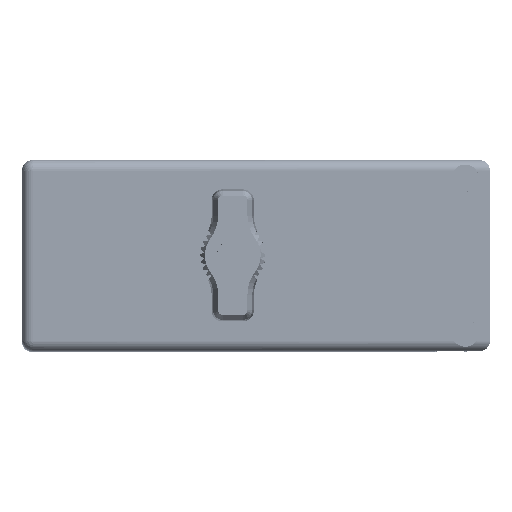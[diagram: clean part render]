
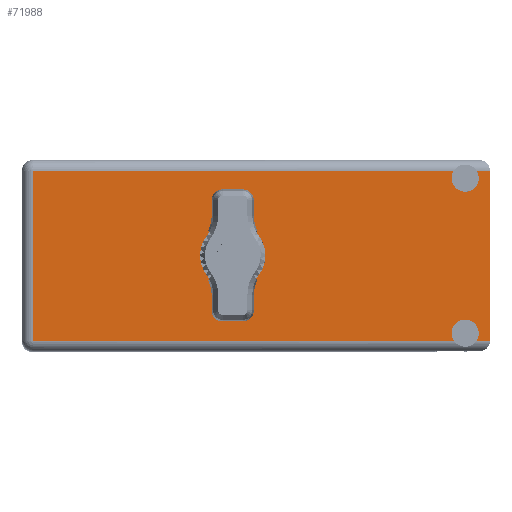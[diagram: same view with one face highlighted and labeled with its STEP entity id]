
A CAD part, top view. The second image highlights one B-rep face of the part: STEP entity #71988.
In plain terms, the highlighted face is planar.
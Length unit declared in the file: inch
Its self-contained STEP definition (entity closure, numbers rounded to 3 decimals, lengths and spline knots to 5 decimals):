
#157 = DIRECTION ( 'NONE',  ( -1., 0., 0. ) ) ;
#240 = AXIS2_PLACEMENT_3D ( 'NONE', #29537, #90201, #157 ) ;
#545 = EDGE_CURVE ( 'NONE', #49202, #39092, #40444, .T. ) ;
#742 = CIRCLE ( 'NONE', #60126, 0.125 ) ;
#1376 = LINE ( 'NONE', #47346, #81972 ) ;
#2965 = ORIENTED_EDGE ( 'NONE', *, *, #45895, .F. ) ;
#4074 = ORIENTED_EDGE ( 'NONE', *, *, #80457, .F. ) ;
#6186 = CARTESIAN_POINT ( 'NONE',  ( 0., 1.675, 0. ) ) ;
#7179 = DIRECTION ( 'NONE',  ( 0., 0., 1. ) ) ;
#8169 = LINE ( 'NONE', #76158, #36929 ) ;
#8355 = DIRECTION ( 'NONE',  ( 0., 0., 1. ) ) ;
#8837 = CARTESIAN_POINT ( 'NONE',  ( 1.499, 1.675, 0.5 ) ) ;
#9008 = VERTEX_POINT ( 'NONE', #22564 ) ;
#10022 = EDGE_CURVE ( 'NONE', #57169, #67750, #8169, .T. ) ;
#12033 = VERTEX_POINT ( 'NONE', #65398 ) ;
#13999 = CARTESIAN_POINT ( 'NONE',  ( -1.359, 1.675, -0.547 ) ) ;
#14849 = FACE_OUTER_BOUND ( 'NONE', #69428, .T. ) ;
#14934 = ORIENTED_EDGE ( 'NONE', *, *, #545, .F. ) ;
#15475 = DIRECTION ( 'NONE',  ( -1., 0., 0. ) ) ;
#17427 = ORIENTED_EDGE ( 'NONE', *, *, #10022, .T. ) ;
#17647 = VERTEX_POINT ( 'NONE', #90620 ) ;
#18313 = LINE ( 'NONE', #78057, #55461 ) ;
#19365 = EDGE_CURVE ( 'NONE', #66767, #9008, #59219, .T. ) ;
#20354 = DIRECTION ( 'NONE',  ( 0., 0., 1. ) ) ;
#22233 = AXIS2_PLACEMENT_3D ( 'NONE', #75167, #61411, #7179 ) ;
#22564 = CARTESIAN_POINT ( 'NONE',  ( -1.289, 1.675, 0.547 ) ) ;
#22662 = FACE_BOUND ( 'NONE', #23826, .T. ) ;
#23826 = EDGE_LOOP ( 'NONE', ( #58635, #71848 ) ) ;
#25578 = CARTESIAN_POINT ( 'NONE',  ( 1.57281, 1.675, -0.547 ) ) ;
#27305 = EDGE_CURVE ( 'NONE', #12033, #66767, #95236, .T. ) ;
#27334 = EDGE_CURVE ( 'NONE', #17647, #52103, #742, .T. ) ;
#27689 = EDGE_CURVE ( 'NONE', #52103, #17647, #45992, .T. ) ;
#27921 = DIRECTION ( 'NONE',  ( 0., 0., 1. ) ) ;
#28502 = DIRECTION ( 'NONE',  ( 0., 1., 0. ) ) ;
#29537 = CARTESIAN_POINT ( 'NONE',  ( -1.359, 1.675, -0.617 ) ) ;
#33603 = CARTESIAN_POINT ( 'NONE',  ( 1.57281, 1.675, 0.547 ) ) ;
#36219 = CARTESIAN_POINT ( 'NONE',  ( 1.499, 1.675, -0.5 ) ) ;
#36795 = CARTESIAN_POINT ( 'NONE',  ( 1.499, 1.675, 0.5 ) ) ;
#36929 = VECTOR ( 'NONE', #15475, 39.37008 ) ;
#36974 = ORIENTED_EDGE ( 'NONE', *, *, #95098, .F. ) ;
#38511 = EDGE_CURVE ( 'NONE', #58646, #67750, #48663, .T. ) ;
#38644 = DIRECTION ( 'NONE',  ( 0., 1., 0. ) ) ;
#39092 = VERTEX_POINT ( 'NONE', #65973 ) ;
#40444 = CIRCLE ( 'NONE', #96788, 0.0875 ) ;
#41297 = AXIS2_PLACEMENT_3D ( 'NONE', #59632, #66966, #52278 ) ;
#41910 = CARTESIAN_POINT ( 'NONE',  ( 1.499, 1.675, -0.4125 ) ) ;
#43825 = DIRECTION ( 'NONE',  ( -1., 0., 0. ) ) ;
#45895 = EDGE_CURVE ( 'NONE', #57169, #48345, #94169, .T. ) ;
#45992 = CIRCLE ( 'NONE', #41297, 0.125 ) ;
#46179 = ORIENTED_EDGE ( 'NONE', *, *, #19365, .T. ) ;
#46536 = EDGE_CURVE ( 'NONE', #56596, #48345, #1376, .T. ) ;
#47346 = CARTESIAN_POINT ( 'NONE',  ( 1.659, 1.675, 0.547 ) ) ;
#48345 = VERTEX_POINT ( 'NONE', #94891 ) ;
#48663 = CIRCLE ( 'NONE', #64315, 0.0875 ) ;
#48972 = EDGE_CURVE ( 'NONE', #9008, #39092, #18313, .T. ) ;
#49202 = VERTEX_POINT ( 'NONE', #73497 ) ;
#50108 = CARTESIAN_POINT ( 'NONE',  ( 0., 1.675, 0.125 ) ) ;
#51509 = ORIENTED_EDGE ( 'NONE', *, *, #27305, .T. ) ;
#52103 = VERTEX_POINT ( 'NONE', #50108 ) ;
#52278 = DIRECTION ( 'NONE',  ( 0., 0., 1. ) ) ;
#53714 = AXIS2_PLACEMENT_3D ( 'NONE', #8837, #38644, #8355 ) ;
#55461 = VECTOR ( 'NONE', #61912, 39.37008 ) ;
#56596 = VERTEX_POINT ( 'NONE', #33603 ) ;
#57169 = VERTEX_POINT ( 'NONE', #80468 ) ;
#58635 = ORIENTED_EDGE ( 'NONE', *, *, #27689, .F. ) ;
#58646 = VERTEX_POINT ( 'NONE', #41910 ) ;
#59219 = LINE ( 'NONE', #89082, #67057 ) ;
#59632 = CARTESIAN_POINT ( 'NONE',  ( 0., 1.675, 0. ) ) ;
#60126 = AXIS2_PLACEMENT_3D ( 'NONE', #6186, #96690, #20354 ) ;
#61411 = DIRECTION ( 'NONE',  ( 0., 1., 0. ) ) ;
#61912 = DIRECTION ( 'NONE',  ( 1., 0., 0. ) ) ;
#62518 = DIRECTION ( 'NONE',  ( 1., 0., 0. ) ) ;
#63637 = VECTOR ( 'NONE', #65753, 39.37008 ) ;
#64315 = AXIS2_PLACEMENT_3D ( 'NONE', #36219, #86667, #71985 ) ;
#65398 = CARTESIAN_POINT ( 'NONE',  ( 1.42519, 1.675, -0.547 ) ) ;
#65753 = DIRECTION ( 'NONE',  ( 0., 0., 1. ) ) ;
#65973 = CARTESIAN_POINT ( 'NONE',  ( 1.42519, 1.675, 0.547 ) ) ;
#66649 = DIRECTION ( 'NONE',  ( 0., 0., 1. ) ) ;
#66716 = PLANE ( 'NONE',  #240 ) ;
#66767 = VERTEX_POINT ( 'NONE', #85494 ) ;
#66966 = DIRECTION ( 'NONE',  ( 0., 1., 0. ) ) ;
#67057 = VECTOR ( 'NONE', #27921, 39.37008 ) ;
#67750 = VERTEX_POINT ( 'NONE', #25578 ) ;
#69428 = EDGE_LOOP ( 'NONE', ( #77994, #14934, #36974, #83985, #2965, #17427, #95449, #4074, #51509, #46179 ) ) ;
#70895 = CIRCLE ( 'NONE', #53714, 0.0875 ) ;
#71848 = ORIENTED_EDGE ( 'NONE', *, *, #27334, .F. ) ;
#71985 = DIRECTION ( 'NONE',  ( 0., 0., 1. ) ) ;
#71988 = ADVANCED_FACE ( 'NONE', ( #22662, #14849 ), #66716, .T. ) ;
#73497 = CARTESIAN_POINT ( 'NONE',  ( 1.499, 1.675, 0.4125 ) ) ;
#75167 = CARTESIAN_POINT ( 'NONE',  ( 1.499, 1.675, -0.5 ) ) ;
#75718 = VECTOR ( 'NONE', #43825, 39.37008 ) ;
#76158 = CARTESIAN_POINT ( 'NONE',  ( -1.359, 1.675, -0.547 ) ) ;
#77994 = ORIENTED_EDGE ( 'NONE', *, *, #48972, .T. ) ;
#78057 = CARTESIAN_POINT ( 'NONE',  ( 1.659, 1.675, 0.547 ) ) ;
#80457 = EDGE_CURVE ( 'NONE', #12033, #58646, #86353, .T. ) ;
#80468 = CARTESIAN_POINT ( 'NONE',  ( 1.659, 1.675, -0.547 ) ) ;
#81972 = VECTOR ( 'NONE', #62518, 39.37008 ) ;
#83985 = ORIENTED_EDGE ( 'NONE', *, *, #46536, .T. ) ;
#85494 = CARTESIAN_POINT ( 'NONE',  ( -1.289, 1.675, -0.547 ) ) ;
#86353 = CIRCLE ( 'NONE', #22233, 0.0875 ) ;
#86667 = DIRECTION ( 'NONE',  ( 0., 1., 0. ) ) ;
#89082 = CARTESIAN_POINT ( 'NONE',  ( -1.289, 1.675, -0.617 ) ) ;
#90201 = DIRECTION ( 'NONE',  ( 0., 1., 0. ) ) ;
#90620 = CARTESIAN_POINT ( 'NONE',  ( 0., 1.675, -0.125 ) ) ;
#94169 = LINE ( 'NONE', #95128, #63637 ) ;
#94891 = CARTESIAN_POINT ( 'NONE',  ( 1.659, 1.675, 0.547 ) ) ;
#95098 = EDGE_CURVE ( 'NONE', #56596, #49202, #70895, .T. ) ;
#95128 = CARTESIAN_POINT ( 'NONE',  ( 1.659, 1.675, 0.617 ) ) ;
#95236 = LINE ( 'NONE', #13999, #75718 ) ;
#95449 = ORIENTED_EDGE ( 'NONE', *, *, #38511, .F. ) ;
#96690 = DIRECTION ( 'NONE',  ( 0., 1., 0. ) ) ;
#96788 = AXIS2_PLACEMENT_3D ( 'NONE', #36795, #28502, #66649 ) ;
